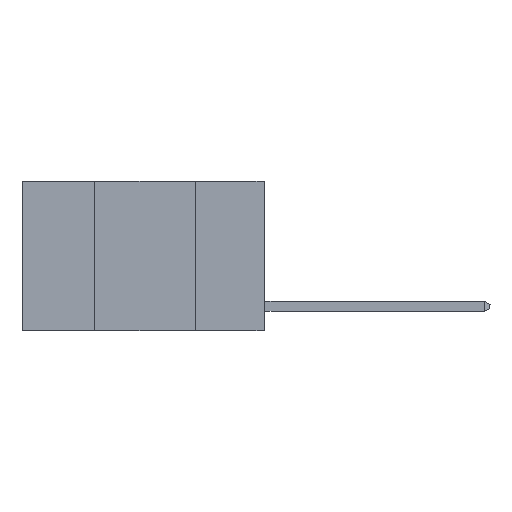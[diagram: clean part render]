
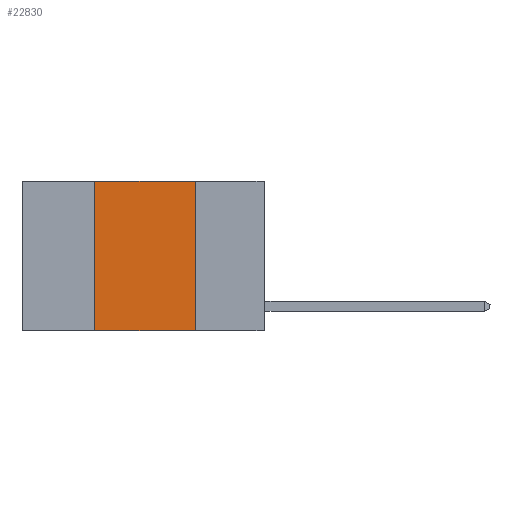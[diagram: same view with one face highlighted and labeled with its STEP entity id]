
A CAD part, left-side view. The second image highlights one B-rep face of the part: STEP entity #22830.
In plain terms, the highlighted planar face has unit normal (-1, 0, 0).
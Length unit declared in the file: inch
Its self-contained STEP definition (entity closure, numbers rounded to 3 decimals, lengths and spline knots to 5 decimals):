
#121 = FACE_OUTER_BOUND ( 'NONE', #6157, .T. ) ;
#537 = VERTEX_POINT ( 'NONE', #12570 ) ;
#725 = CARTESIAN_POINT ( 'NONE',  ( 0., 0.6, -0.37 ) ) ;
#1147 = VERTEX_POINT ( 'NONE', #10490 ) ;
#3288 = VECTOR ( 'NONE', #4413, 39.37008 ) ;
#3487 = EDGE_CURVE ( 'NONE', #20650, #12352, #7328, .T. ) ;
#3961 = LINE ( 'NONE', #19859, #23045 ) ;
#4113 = DIRECTION ( 'NONE',  ( 0., -1., 0. ) ) ;
#4413 = DIRECTION ( 'NONE',  ( 0., -1., 0. ) ) ;
#4716 = AXIS2_PLACEMENT_3D ( 'NONE', #19428, #12470, #10535 ) ;
#6157 = EDGE_LOOP ( 'NONE', ( #12231, #24354, #19889, #17274 ) ) ;
#6888 = DIRECTION ( 'NONE',  ( 0., 0., -1. ) ) ;
#7328 = LINE ( 'NONE', #18379, #9741 ) ;
#8046 = EDGE_CURVE ( 'NONE', #1147, #20650, #19089, .T. ) ;
#8347 = LINE ( 'NONE', #725, #3288 ) ;
#8354 = PLANE ( 'NONE',  #4716 ) ;
#9741 = VECTOR ( 'NONE', #6888, 39.37008 ) ;
#9954 = CARTESIAN_POINT ( 'NONE',  ( 0., 0.17, -0.37 ) ) ;
#10490 = CARTESIAN_POINT ( 'NONE',  ( 0., 0.42, 0. ) ) ;
#10535 = DIRECTION ( 'NONE',  ( 0., 0., -1. ) ) ;
#11678 = VECTOR ( 'NONE', #4113, 39.37008 ) ;
#12231 = ORIENTED_EDGE ( 'NONE', *, *, #3487, .F. ) ;
#12352 = VERTEX_POINT ( 'NONE', #9954 ) ;
#12470 = DIRECTION ( 'NONE',  ( 1., 0., 0. ) ) ;
#12570 = CARTESIAN_POINT ( 'NONE',  ( 0., 0.42, -0.37 ) ) ;
#14354 = EDGE_CURVE ( 'NONE', #537, #1147, #3961, .T. ) ;
#15553 = CARTESIAN_POINT ( 'NONE',  ( 0., 0.6, 0. ) ) ;
#15960 = EDGE_CURVE ( 'NONE', #537, #12352, #8347, .T. ) ;
#17274 = ORIENTED_EDGE ( 'NONE', *, *, #15960, .T. ) ;
#18379 = CARTESIAN_POINT ( 'NONE',  ( 0., 0.17, 0. ) ) ;
#19089 = LINE ( 'NONE', #15553, #11678 ) ;
#19428 = CARTESIAN_POINT ( 'NONE',  ( 0., 0.6, 0. ) ) ;
#19859 = CARTESIAN_POINT ( 'NONE',  ( 0., 0.42, 0. ) ) ;
#19889 = ORIENTED_EDGE ( 'NONE', *, *, #14354, .F. ) ;
#20650 = VERTEX_POINT ( 'NONE', #21338 ) ;
#21338 = CARTESIAN_POINT ( 'NONE',  ( 0., 0.17, 0. ) ) ;
#22830 = ADVANCED_FACE ( 'NONE', ( #121 ), #8354, .F. ) ;
#23045 = VECTOR ( 'NONE', #23688, 39.37008 ) ;
#23688 = DIRECTION ( 'NONE',  ( 0., 0., 1. ) ) ;
#24354 = ORIENTED_EDGE ( 'NONE', *, *, #8046, .F. ) ;
